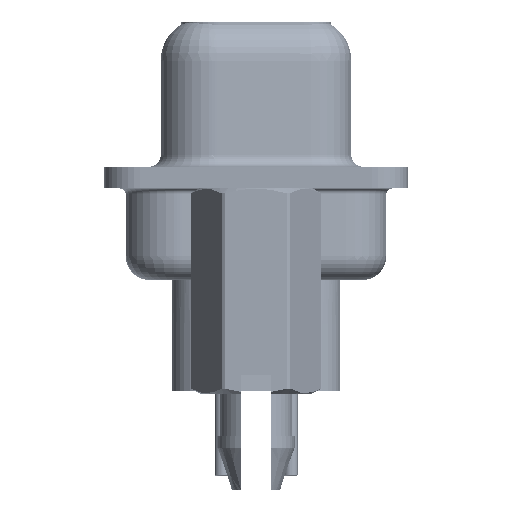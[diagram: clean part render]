
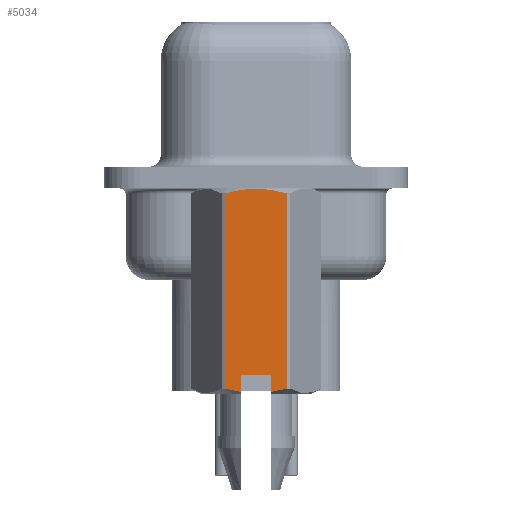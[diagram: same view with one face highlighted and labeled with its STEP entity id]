
A CAD part, left-side view. The second image highlights one B-rep face of the part: STEP entity #5034.
In plain terms, the highlighted planar face has unit normal (-1, 0, 0).
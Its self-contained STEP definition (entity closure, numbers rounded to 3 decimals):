
#143 = VECTOR ( 'NONE', #11544, 1000. ) ;
#314 = DIRECTION ( 'NONE',  ( 0., 0., -1. ) ) ;
#446 = EDGE_CURVE ( 'NONE', #43125, #27517, #7418, .T. ) ;
#506 = CARTESIAN_POINT ( 'NONE',  ( -2.381, 1.273, -0.652 ) ) ;
#571 = CARTESIAN_POINT ( 'NONE',  ( -2.381, -1.375, 7.399 ) ) ;
#1591 = EDGE_CURVE ( 'NONE', #5006, #17540, #33424, .T. ) ;
#3879 = PLANE ( 'NONE',  #25024 ) ;
#4283 = CARTESIAN_POINT ( 'NONE',  ( -2.381, 0.215, -0.468 ) ) ;
#4540 = CARTESIAN_POINT ( 'NONE',  ( -2.381, -1.06, -8.806 ) ) ;
#5006 = VERTEX_POINT ( 'NONE', #42110 ) ;
#5034 = ADVANCED_FACE ( 'NONE', ( #39503 ), #3879, .T. ) ;
#7418 = LINE ( 'NONE', #8115, #22586 ) ;
#7632 = CARTESIAN_POINT ( 'NONE',  ( -2.381, -0.625, -8.2 ) ) ;
#7846 = EDGE_CURVE ( 'NONE', #41898, #26540, #46280, .T. ) ;
#8096 = CARTESIAN_POINT ( 'NONE',  ( -2.381, -0.842, -8.854 ) ) ;
#8115 = CARTESIAN_POINT ( 'NONE',  ( -2.381, 0.625, -8.2 ) ) ;
#9535 = EDGE_CURVE ( 'NONE', #11336, #41898, #45280, .T. ) ;
#9817 = CARTESIAN_POINT ( 'NONE',  ( -2.381, -0.625, -8.2 ) ) ;
#10289 = CARTESIAN_POINT ( 'NONE',  ( -2.381, 0., -0.468 ) ) ;
#10466 = CARTESIAN_POINT ( 'NONE',  ( -2.381, 0.432, -0.485 ) ) ;
#10502 = CARTESIAN_POINT ( 'NONE',  ( -2.381, 0.625, -8.885 ) ) ;
#10672 = VERTEX_POINT ( 'NONE', #35517 ) ;
#10876 = EDGE_CURVE ( 'NONE', #10672, #11336, #16955, .T. ) ;
#11299 = LINE ( 'NONE', #21995, #143 ) ;
#11336 = VERTEX_POINT ( 'NONE', #10289 ) ;
#11544 = DIRECTION ( 'NONE',  ( 0., 1., 0. ) ) ;
#11801 = VECTOR ( 'NONE', #17819, 1000. ) ;
#11884 = CARTESIAN_POINT ( 'NONE',  ( -2.381, -1.273, -8.748 ) ) ;
#12428 = EDGE_CURVE ( 'NONE', #45562, #5006, #20252, .T. ) ;
#14608 = B_SPLINE_CURVE_WITH_KNOTS ( 'NONE', 3,
 ( #29241, #22349, #36155, #10502 ),
 .UNSPECIFIED., .F., .F.,
 ( 4, 4 ),
 ( 0.001, 0.002 ),
 .UNSPECIFIED. ) ;
#15060 = CARTESIAN_POINT ( 'NONE',  ( -2.381, 1.273, -0.652 ) ) ;
#15880 = ORIENTED_EDGE ( 'NONE', *, *, #10876, .T. ) ;
#16133 = EDGE_LOOP ( 'NONE', ( #23670, #21046, #39110, #33790, #34411, #15880, #25263, #42130, #27558 ) ) ;
#16955 = B_SPLINE_CURVE_WITH_KNOTS ( 'NONE', 3,
 ( #36689, #29319, #40720, #19091, #37411, #43801 ),
 .UNSPECIFIED., .F., .F.,
 ( 4, 2, 4 ),
 ( 0.003, 0.003, 0.004 ),
 .UNSPECIFIED. ) ;
#17540 = VERTEX_POINT ( 'NONE', #46816 ) ;
#17819 = DIRECTION ( 'NONE',  ( 0., 0., 1. ) ) ;
#19091 = CARTESIAN_POINT ( 'NONE',  ( -2.381, -0.428, -0.485 ) ) ;
#20252 = LINE ( 'NONE', #9817, #44572 ) ;
#21046 = ORIENTED_EDGE ( 'NONE', *, *, #34460, .F. ) ;
#21681 = DIRECTION ( 'NONE',  ( -1., 0., 0. ) ) ;
#21995 = CARTESIAN_POINT ( 'NONE',  ( -2.381, -0.625, -8.2 ) ) ;
#22051 = DIRECTION ( 'NONE',  ( 0., 0., -1. ) ) ;
#22312 = CARTESIAN_POINT ( 'NONE',  ( -2.381, 0.858, -0.55 ) ) ;
#22349 = CARTESIAN_POINT ( 'NONE',  ( -2.381, 1.06, -8.806 ) ) ;
#22586 = VECTOR ( 'NONE', #314, 1000. ) ;
#23670 = ORIENTED_EDGE ( 'NONE', *, *, #446, .F. ) ;
#25024 = AXIS2_PLACEMENT_3D ( 'NONE', #571, #21681, #25944 ) ;
#25263 = ORIENTED_EDGE ( 'NONE', *, *, #9535, .T. ) ;
#25647 = CARTESIAN_POINT ( 'NONE',  ( -2.381, 0., -0.468 ) ) ;
#25944 = DIRECTION ( 'NONE',  ( 0., 0., 1. ) ) ;
#26540 = VERTEX_POINT ( 'NONE', #44263 ) ;
#27517 = VERTEX_POINT ( 'NONE', #30202 ) ;
#27558 = ORIENTED_EDGE ( 'NONE', *, *, #37180, .T. ) ;
#28021 = LINE ( 'NONE', #40142, #11801 ) ;
#28234 = CARTESIAN_POINT ( 'NONE',  ( -2.381, 1.273, 0.581 ) ) ;
#29241 = CARTESIAN_POINT ( 'NONE',  ( -2.381, 1.273, -8.748 ) ) ;
#29319 = CARTESIAN_POINT ( 'NONE',  ( -2.381, -1.065, -0.596 ) ) ;
#30202 = CARTESIAN_POINT ( 'NONE',  ( -2.381, 0.625, -8.885 ) ) ;
#30250 = EDGE_CURVE ( 'NONE', #17540, #10672, #28021, .T. ) ;
#33424 = B_SPLINE_CURVE_WITH_KNOTS ( 'NONE', 3,
 ( #44421, #8096, #4540, #11884 ),
 .UNSPECIFIED., .F., .F.,
 ( 4, 4 ),
 ( 0.003, 0.004 ),
 .UNSPECIFIED. ) ;
#33790 = ORIENTED_EDGE ( 'NONE', *, *, #1591, .T. ) ;
#34382 = CARTESIAN_POINT ( 'NONE',  ( -2.381, 0.625, -8.2 ) ) ;
#34411 = ORIENTED_EDGE ( 'NONE', *, *, #30250, .T. ) ;
#34460 = EDGE_CURVE ( 'NONE', #45562, #43125, #11299, .T. ) ;
#35517 = CARTESIAN_POINT ( 'NONE',  ( -2.381, -1.273, -0.652 ) ) ;
#36155 = CARTESIAN_POINT ( 'NONE',  ( -2.381, 0.845, -8.853 ) ) ;
#36689 = CARTESIAN_POINT ( 'NONE',  ( -2.381, -1.273, -0.652 ) ) ;
#37180 = EDGE_CURVE ( 'NONE', #26540, #27517, #14608, .T. ) ;
#37324 = VECTOR ( 'NONE', #22051, 1000. ) ;
#37411 = CARTESIAN_POINT ( 'NONE',  ( -2.381, -0.215, -0.468 ) ) ;
#37867 = DIRECTION ( 'NONE',  ( 0., 0., -1. ) ) ;
#39110 = ORIENTED_EDGE ( 'NONE', *, *, #12428, .T. ) ;
#39503 = FACE_OUTER_BOUND ( 'NONE', #16133, .T. ) ;
#39680 = CARTESIAN_POINT ( 'NONE',  ( -2.381, 1.066, -0.596 ) ) ;
#40142 = CARTESIAN_POINT ( 'NONE',  ( -2.381, -1.273, 0.581 ) ) ;
#40720 = CARTESIAN_POINT ( 'NONE',  ( -2.381, -0.853, -0.549 ) ) ;
#41898 = VERTEX_POINT ( 'NONE', #15060 ) ;
#42110 = CARTESIAN_POINT ( 'NONE',  ( -2.381, -0.625, -8.885 ) ) ;
#42130 = ORIENTED_EDGE ( 'NONE', *, *, #7846, .T. ) ;
#43125 = VERTEX_POINT ( 'NONE', #34382 ) ;
#43801 = CARTESIAN_POINT ( 'NONE',  ( -2.381, 0., -0.468 ) ) ;
#44263 = CARTESIAN_POINT ( 'NONE',  ( -2.381, 1.273, -8.748 ) ) ;
#44421 = CARTESIAN_POINT ( 'NONE',  ( -2.381, -0.625, -8.885 ) ) ;
#44572 = VECTOR ( 'NONE', #37867, 1000. ) ;
#45280 = B_SPLINE_CURVE_WITH_KNOTS ( 'NONE', 3,
 ( #25647, #4283, #10466, #22312, #39680, #506 ),
 .UNSPECIFIED., .F., .F.,
 ( 4, 2, 4 ),
 ( 0.004, 0.004, 0.005 ),
 .UNSPECIFIED. ) ;
#45562 = VERTEX_POINT ( 'NONE', #7632 ) ;
#46280 = LINE ( 'NONE', #28234, #37324 ) ;
#46816 = CARTESIAN_POINT ( 'NONE',  ( -2.381, -1.273, -8.748 ) ) ;
